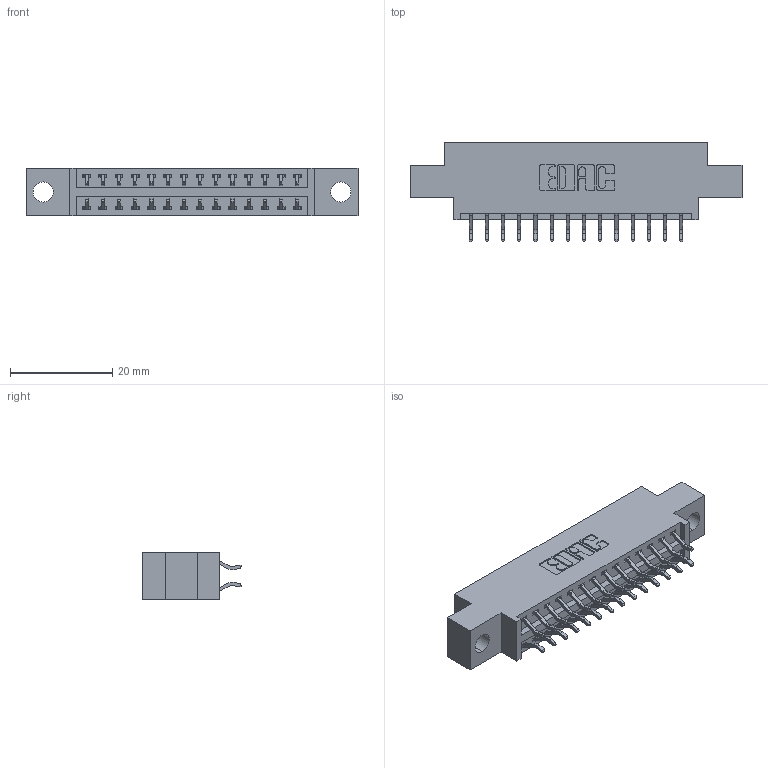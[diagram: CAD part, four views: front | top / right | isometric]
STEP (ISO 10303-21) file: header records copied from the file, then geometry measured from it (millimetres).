
FILE_DESCRIPTION (( 'STEP AP203' ), '1' );
FILE_NAME ('346-028-556-804.STEP', '2022-05-19T05:11:39', ( '' ), ( '' ), 'SwSTEP 2.0', 'SolidWorks 2020', '' );
FILE_SCHEMA (( 'CONFIG_CONTROL_DESIGN' ));
Length unit declared in the file: inch
Products named in the file (3): 345-292-001_556 Tail; 346-028-556-804; 346 Part_0.170 Offset - 0.156 Dia-TH
Assembly tree (29 placements, depth 2):
  346-028-556-804
    346 Part_0.170 Offset - 0.156 Dia-TH
    345-292-001_556 Tail  x28
Bounding box: 65.02 x 19.57 x 9.4 mm (x, y, z)
Volume: 5861.5 mm3; surface area: 7618.4 mm2
Topology: 29 solids, 29 shells, 1764 faces, 5221 edges, 3442 vertices
Faces by surface type: plane 1186, cylinder 578
Entity records: 13677 total; most frequent: CARTESIAN_POINT 2314, ORIENTED_EDGE 2234, DIRECTION 2077, EDGE_CURVE 1117, VECTOR 921, LINE 921, VERTEX_POINT 742, AXIS2_PLACEMENT_3D 578
